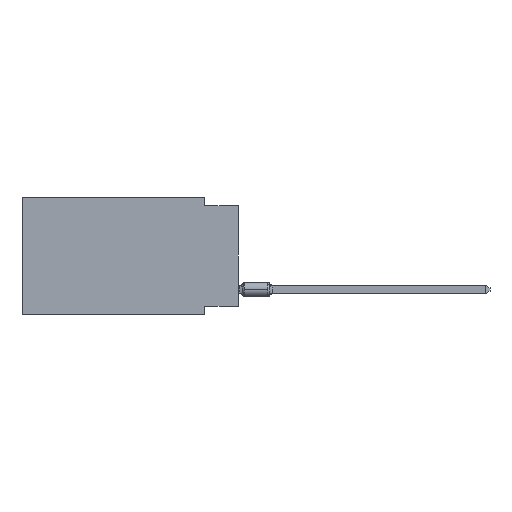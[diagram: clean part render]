
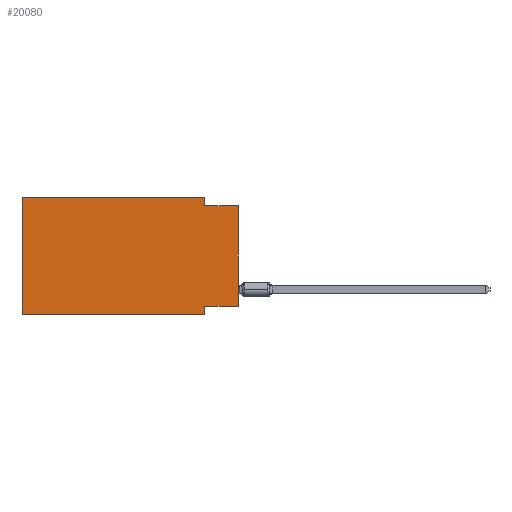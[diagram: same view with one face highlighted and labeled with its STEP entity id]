
A CAD part, left-side view. The second image highlights one B-rep face of the part: STEP entity #20080.
In plain terms, the highlighted planar face has unit normal (-1, 0, 0).
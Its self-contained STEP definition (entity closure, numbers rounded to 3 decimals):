
#1163 = VECTOR ( 'NONE', #32338, 1000. ) ;
#1810 = EDGE_CURVE ( 'NONE', #33553, #27659, #12063, .T. ) ;
#3721 = EDGE_CURVE ( 'NONE', #26808, #20828, #36692, .T. ) ;
#4124 = AXIS2_PLACEMENT_3D ( 'NONE', #8015, #14642, #13777 ) ;
#4233 = EDGE_CURVE ( 'NONE', #38034, #13750, #34179, .T. ) ;
#4684 = VERTEX_POINT ( 'NONE', #30400 ) ;
#4998 = CARTESIAN_POINT ( 'NONE',  ( 0., 0., -8.255 ) ) ;
#5437 = CARTESIAN_POINT ( 'NONE',  ( 0., 2.54, 0. ) ) ;
#5845 = VECTOR ( 'NONE', #22596, 1000. ) ;
#6845 = CARTESIAN_POINT ( 'NONE',  ( 0., 0., 0. ) ) ;
#7708 = EDGE_CURVE ( 'NONE', #33553, #26808, #27411, .T. ) ;
#8015 = CARTESIAN_POINT ( 'NONE',  ( 0., 16.383, 0. ) ) ;
#8275 = VECTOR ( 'NONE', #16410, 1000. ) ;
#8483 = DIRECTION ( 'NONE',  ( 0., 0., -1. ) ) ;
#10186 = CARTESIAN_POINT ( 'NONE',  ( 0., 16.383, 0. ) ) ;
#12063 = LINE ( 'NONE', #18893, #1163 ) ;
#12157 = CARTESIAN_POINT ( 'NONE',  ( 0., 2.54, 0. ) ) ;
#12339 = EDGE_CURVE ( 'NONE', #26195, #13750, #22435, .T. ) ;
#13530 = ORIENTED_EDGE ( 'NONE', *, *, #3721, .F. ) ;
#13750 = VERTEX_POINT ( 'NONE', #38343 ) ;
#13777 = DIRECTION ( 'NONE',  ( 0., 0., -1. ) ) ;
#13806 = CARTESIAN_POINT ( 'NONE',  ( 0., 16.383, -8.89 ) ) ;
#13965 = CARTESIAN_POINT ( 'NONE',  ( 0., 16.383, 0. ) ) ;
#14642 = DIRECTION ( 'NONE',  ( 1., 0., 0. ) ) ;
#15144 = ORIENTED_EDGE ( 'NONE', *, *, #1810, .T. ) ;
#16344 = ORIENTED_EDGE ( 'NONE', *, *, #31752, .F. ) ;
#16410 = DIRECTION ( 'NONE',  ( 0., -1., 0. ) ) ;
#18220 = EDGE_CURVE ( 'NONE', #20828, #26195, #32208, .T. ) ;
#18329 = ORIENTED_EDGE ( 'NONE', *, *, #18220, .F. ) ;
#18332 = DIRECTION ( 'NONE',  ( 0., 0., -1. ) ) ;
#18893 = CARTESIAN_POINT ( 'NONE',  ( 0., 16.383, -8.89 ) ) ;
#19322 = VECTOR ( 'NONE', #32364, 1000. ) ;
#19705 = CARTESIAN_POINT ( 'NONE',  ( 0., 16.383, 0. ) ) ;
#19723 = CARTESIAN_POINT ( 'NONE',  ( 0., 0., -8.255 ) ) ;
#20080 = ADVANCED_FACE ( 'NONE', ( #20817 ), #41313, .F. ) ;
#20588 = ORIENTED_EDGE ( 'NONE', *, *, #29957, .F. ) ;
#20817 = FACE_OUTER_BOUND ( 'NONE', #43394, .T. ) ;
#20828 = VERTEX_POINT ( 'NONE', #5437 ) ;
#22435 = LINE ( 'NONE', #42287, #19322 ) ;
#22596 = DIRECTION ( 'NONE',  ( 0., 1., 0. ) ) ;
#23227 = DIRECTION ( 'NONE',  ( 0., 0., 1. ) ) ;
#24053 = DIRECTION ( 'NONE',  ( 0., 0., 1. ) ) ;
#25169 = ORIENTED_EDGE ( 'NONE', *, *, #12339, .F. ) ;
#26195 = VERTEX_POINT ( 'NONE', #28341 ) ;
#26808 = VERTEX_POINT ( 'NONE', #10186 ) ;
#27046 = LINE ( 'NONE', #28133, #35400 ) ;
#27411 = LINE ( 'NONE', #13965, #34507 ) ;
#27659 = VERTEX_POINT ( 'NONE', #33216 ) ;
#28133 = CARTESIAN_POINT ( 'NONE',  ( 0., 2.54, -8.89 ) ) ;
#28303 = ORIENTED_EDGE ( 'NONE', *, *, #4233, .T. ) ;
#28341 = CARTESIAN_POINT ( 'NONE',  ( 0., 2.54, -0.635 ) ) ;
#29957 = EDGE_CURVE ( 'NONE', #38034, #4684, #39579, .T. ) ;
#30400 = CARTESIAN_POINT ( 'NONE',  ( 0., 2.54, -8.255 ) ) ;
#31752 = EDGE_CURVE ( 'NONE', #4684, #27659, #27046, .T. ) ;
#32208 = LINE ( 'NONE', #12157, #38544 ) ;
#32338 = DIRECTION ( 'NONE',  ( 0., -1., 0. ) ) ;
#32364 = DIRECTION ( 'NONE',  ( 0., -1., 0. ) ) ;
#33216 = CARTESIAN_POINT ( 'NONE',  ( 0., 2.54, -8.89 ) ) ;
#33553 = VERTEX_POINT ( 'NONE', #13806 ) ;
#34179 = LINE ( 'NONE', #6845, #34378 ) ;
#34378 = VECTOR ( 'NONE', #24053, 1000. ) ;
#34507 = VECTOR ( 'NONE', #23227, 1000. ) ;
#35400 = VECTOR ( 'NONE', #8483, 1000. ) ;
#36692 = LINE ( 'NONE', #19705, #8275 ) ;
#37978 = ORIENTED_EDGE ( 'NONE', *, *, #7708, .F. ) ;
#38034 = VERTEX_POINT ( 'NONE', #4998 ) ;
#38343 = CARTESIAN_POINT ( 'NONE',  ( 0., 0., -0.635 ) ) ;
#38544 = VECTOR ( 'NONE', #18332, 1000. ) ;
#39579 = LINE ( 'NONE', #19723, #5845 ) ;
#41313 = PLANE ( 'NONE',  #4124 ) ;
#42287 = CARTESIAN_POINT ( 'NONE',  ( 0., 0., -0.635 ) ) ;
#43394 = EDGE_LOOP ( 'NONE', ( #28303, #25169, #18329, #13530, #37978, #15144, #16344, #20588 ) ) ;
